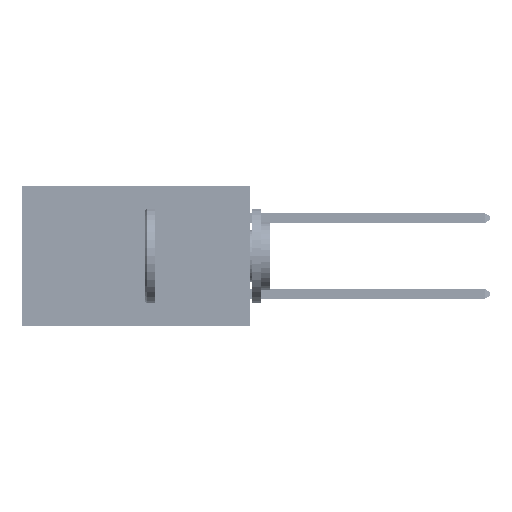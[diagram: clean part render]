
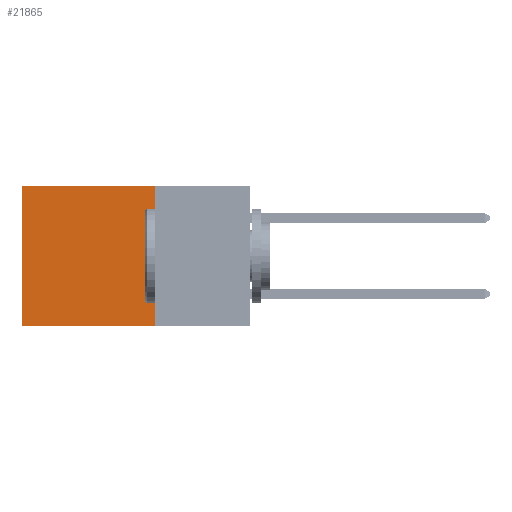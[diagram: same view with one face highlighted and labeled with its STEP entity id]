
A CAD part, left-side view. The second image highlights one B-rep face of the part: STEP entity #21865.
In plain terms, the highlighted planar face has unit normal (-1, 0, 0).
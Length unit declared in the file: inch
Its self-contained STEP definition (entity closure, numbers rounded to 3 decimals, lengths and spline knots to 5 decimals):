
#4039 = AXIS2_PLACEMENT_3D ( 'NONE', #48913, #21901, #49576 ) ;
#5531 = LINE ( 'NONE', #23396, #13469 ) ;
#6116 = PLANE ( 'NONE',  #4039 ) ;
#6330 = LINE ( 'NONE', #25416, #33757 ) ;
#7501 = ORIENTED_EDGE ( 'NONE', *, *, #8510, .F. ) ;
#8510 = EDGE_CURVE ( 'NONE', #46550, #17831, #5531, .T. ) ;
#11344 = EDGE_CURVE ( 'NONE', #17831, #15000, #40626, .T. ) ;
#12556 = ORIENTED_EDGE ( 'NONE', *, *, #45135, .T. ) ;
#12619 = CARTESIAN_POINT ( 'NONE',  ( 0.2875, 0.25, 0. ) ) ;
#13469 = VECTOR ( 'NONE', #42798, 39.37008 ) ;
#14440 = ORIENTED_EDGE ( 'NONE', *, *, #38043, .T. ) ;
#15000 = VERTEX_POINT ( 'NONE', #40268 ) ;
#17058 = EDGE_LOOP ( 'NONE', ( #14440, #25471, #7501, #12556 ) ) ;
#17831 = VERTEX_POINT ( 'NONE', #47109 ) ;
#21865 = ADVANCED_FACE ( 'NONE', ( #43035 ), #6116, .F. ) ;
#21901 = DIRECTION ( 'NONE',  ( 1., 0., 0. ) ) ;
#22244 = VECTOR ( 'NONE', #26239, 39.37008 ) ;
#23396 = CARTESIAN_POINT ( 'NONE',  ( 0.2875, 0.25, 0. ) ) ;
#25416 = CARTESIAN_POINT ( 'NONE',  ( 0.2875, 0.6, 0. ) ) ;
#25471 = ORIENTED_EDGE ( 'NONE', *, *, #11344, .F. ) ;
#26239 = DIRECTION ( 'NONE',  ( 0., 1., 0. ) ) ;
#28364 = LINE ( 'NONE', #44508, #32632 ) ;
#29011 = DIRECTION ( 'NONE',  ( 0., 0., -1. ) ) ;
#32632 = VECTOR ( 'NONE', #32878, 39.37008 ) ;
#32878 = DIRECTION ( 'NONE',  ( 0., 1., 0. ) ) ;
#33757 = VECTOR ( 'NONE', #29011, 39.37008 ) ;
#33942 = CARTESIAN_POINT ( 'NONE',  ( 0.2875, 0.25, -0.37 ) ) ;
#38043 = EDGE_CURVE ( 'NONE', #38735, #15000, #6330, .T. ) ;
#38735 = VERTEX_POINT ( 'NONE', #45509 ) ;
#40268 = CARTESIAN_POINT ( 'NONE',  ( 0.2875, 0.6, -0.37 ) ) ;
#40626 = LINE ( 'NONE', #33942, #22244 ) ;
#42798 = DIRECTION ( 'NONE',  ( 0., 0., -1. ) ) ;
#43035 = FACE_OUTER_BOUND ( 'NONE', #17058, .T. ) ;
#44508 = CARTESIAN_POINT ( 'NONE',  ( 0.2875, 0.25, 0. ) ) ;
#45135 = EDGE_CURVE ( 'NONE', #46550, #38735, #28364, .T. ) ;
#45509 = CARTESIAN_POINT ( 'NONE',  ( 0.2875, 0.6, 0. ) ) ;
#46550 = VERTEX_POINT ( 'NONE', #12619 ) ;
#47109 = CARTESIAN_POINT ( 'NONE',  ( 0.2875, 0.25, -0.37 ) ) ;
#48913 = CARTESIAN_POINT ( 'NONE',  ( 0.2875, 0.25, 0. ) ) ;
#49576 = DIRECTION ( 'NONE',  ( 0., 0., -1. ) ) ;
